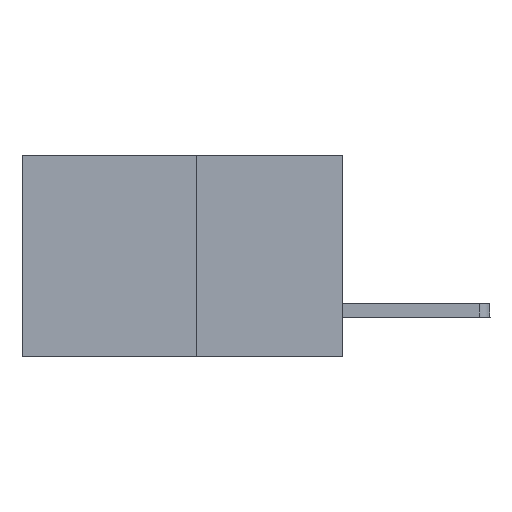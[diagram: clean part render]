
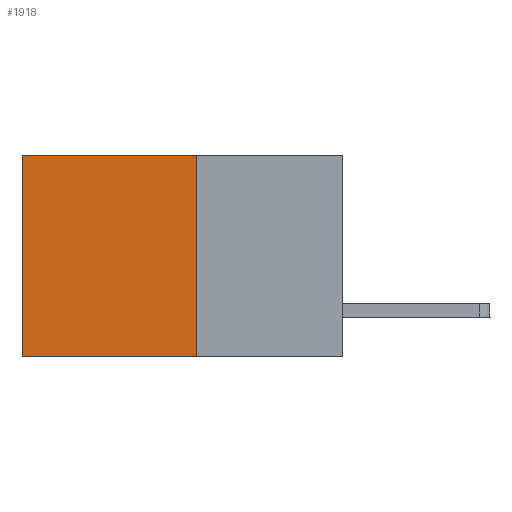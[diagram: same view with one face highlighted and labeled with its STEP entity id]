
A CAD part, left-side view. The second image highlights one B-rep face of the part: STEP entity #1918.
In plain terms, the highlighted planar face has unit normal (-1, 0, 0).
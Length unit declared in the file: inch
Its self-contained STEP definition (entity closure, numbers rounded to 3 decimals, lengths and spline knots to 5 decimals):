
#314 = VERTEX_POINT ( 'NONE', #3601 ) ;
#999 = CARTESIAN_POINT ( 'NONE',  ( 0.277, 0.27, -0.37 ) ) ;
#1344 = CARTESIAN_POINT ( 'NONE',  ( 0.277, 0.27, 0. ) ) ;
#1439 = DIRECTION ( 'NONE',  ( 0., 1., 0. ) ) ;
#1498 = DIRECTION ( 'NONE',  ( 0., 0., -1. ) ) ;
#1728 = DIRECTION ( 'NONE',  ( 0., 0., -1. ) ) ;
#1918 = ADVANCED_FACE ( 'NONE', ( #6982 ), #10427, .F. ) ;
#2216 = VECTOR ( 'NONE', #3538, 39.37008 ) ;
#2290 = VECTOR ( 'NONE', #5557, 39.37008 ) ;
#2711 = ORIENTED_EDGE ( 'NONE', *, *, #5409, .F. ) ;
#3538 = DIRECTION ( 'NONE',  ( 0., 0., -1. ) ) ;
#3601 = CARTESIAN_POINT ( 'NONE',  ( 0.277, 0.27, 0. ) ) ;
#3939 = VERTEX_POINT ( 'NONE', #5382 ) ;
#4188 = ORIENTED_EDGE ( 'NONE', *, *, #9533, .F. ) ;
#4258 = DIRECTION ( 'NONE',  ( 1., 0., 0. ) ) ;
#4268 = CARTESIAN_POINT ( 'NONE',  ( 0.277, 0.27, -0.37 ) ) ;
#4863 = ORIENTED_EDGE ( 'NONE', *, *, #6551, .T. ) ;
#4889 = EDGE_CURVE ( 'NONE', #314, #3939, #8830, .T. ) ;
#5031 = LINE ( 'NONE', #5806, #9067 ) ;
#5316 = VECTOR ( 'NONE', #1498, 39.37008 ) ;
#5382 = CARTESIAN_POINT ( 'NONE',  ( 0.277, 0.59, 0. ) ) ;
#5409 = EDGE_CURVE ( 'NONE', #8576, #5947, #5031, .T. ) ;
#5557 = DIRECTION ( 'NONE',  ( 0., 1., 0. ) ) ;
#5806 = CARTESIAN_POINT ( 'NONE',  ( 0.277, 0.27, -0.37 ) ) ;
#5903 = CARTESIAN_POINT ( 'NONE',  ( 0.277, 0.59, -0.37 ) ) ;
#5947 = VERTEX_POINT ( 'NONE', #5903 ) ;
#6371 = CARTESIAN_POINT ( 'NONE',  ( 0.277, 0.27, -0.37 ) ) ;
#6551 = EDGE_CURVE ( 'NONE', #3939, #5947, #8210, .T. ) ;
#6982 = FACE_OUTER_BOUND ( 'NONE', #11027, .T. ) ;
#7369 = CARTESIAN_POINT ( 'NONE',  ( 0.277, 0.59, -0.37 ) ) ;
#7586 = ORIENTED_EDGE ( 'NONE', *, *, #4889, .T. ) ;
#8210 = LINE ( 'NONE', #7369, #5316 ) ;
#8576 = VERTEX_POINT ( 'NONE', #6371 ) ;
#8830 = LINE ( 'NONE', #1344, #2290 ) ;
#8851 = AXIS2_PLACEMENT_3D ( 'NONE', #999, #4258, #1728 ) ;
#9067 = VECTOR ( 'NONE', #1439, 39.37008 ) ;
#9264 = LINE ( 'NONE', #4268, #2216 ) ;
#9533 = EDGE_CURVE ( 'NONE', #314, #8576, #9264, .T. ) ;
#10427 = PLANE ( 'NONE',  #8851 ) ;
#11027 = EDGE_LOOP ( 'NONE', ( #4863, #2711, #4188, #7586 ) ) ;
